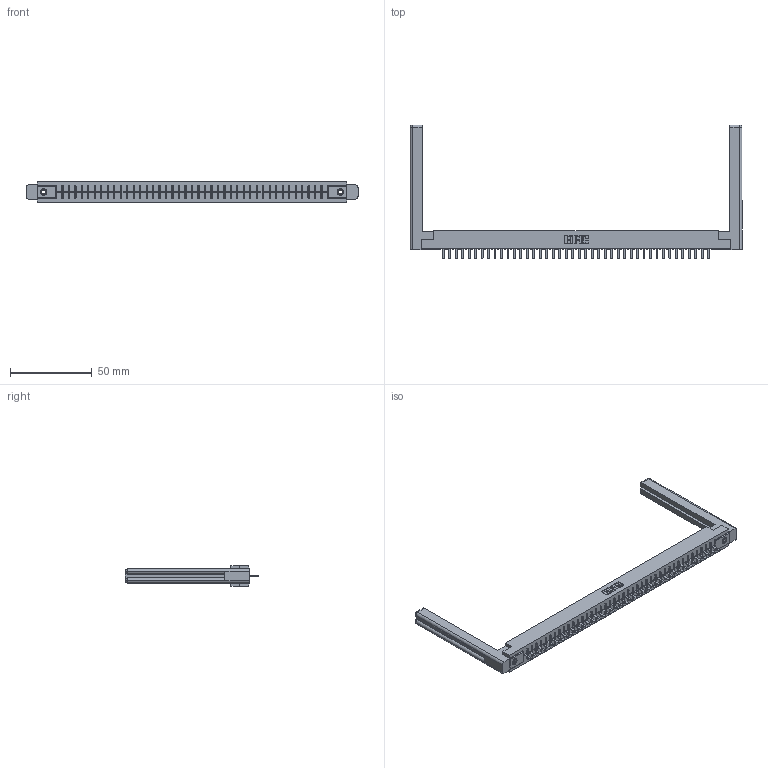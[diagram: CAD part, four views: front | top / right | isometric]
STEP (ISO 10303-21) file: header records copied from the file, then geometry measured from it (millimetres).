
FILE_DESCRIPTION (( 'STEP AP203' ), '1' );
FILE_NAME ('316-042-520-158.STEP', '2018-07-31T05:49:20', ( '' ), ( '' ), 'SwSTEP 2.0', 'SolidWorks 2016', '' );
FILE_SCHEMA (( 'CONFIG_CONTROL_DESIGN' ));
Length unit declared in the file: inch
Products named in the file (5): 306-290-001_120; 345-250-001_345-250-001-102; 307-220-058; 316-042-520-158; 306 Part_.156 Dia
Assembly tree (47 placements, depth 2):
  316-042-520-158
    306 Part_.156 Dia
    306-290-001_120  x42
    345-250-001_345-250-001-102  x2
    307-220-058  x2
Bounding box: 203.05 x 81.76 x 12.7 mm (x, y, z)
Volume: 29540.7 mm3; surface area: 28191.1 mm2
Topology: 47 solids, 47 shells, 3198 faces, 8944 edges, 5724 vertices
Faces by surface type: plane 2126, cylinder 880, sphere 168, cone 12, torus 12
Entity records: 41756 total; most frequent: CARTESIAN_POINT 7020, ORIENTED_EDGE 6902, DIRECTION 6877, EDGE_CURVE 3451, VECTOR 2695, LINE 2695, VERTEX_POINT 2180, AXIS2_PLACEMENT_3D 2091
